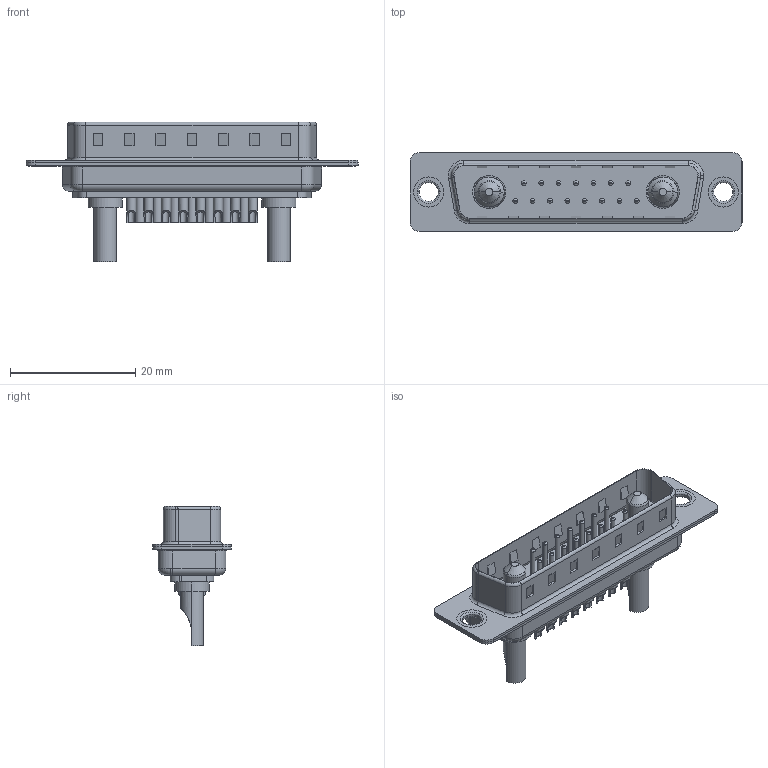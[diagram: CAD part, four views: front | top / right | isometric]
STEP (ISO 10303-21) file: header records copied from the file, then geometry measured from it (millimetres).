
FILE_DESCRIPTION (( 'STEP AP203' ), '1' );
FILE_NAME ('627-17W2222-2N1.STEP', '2019-05-27T14:13:00', ( '' ), ( '' ), 'SwSTEP 2.0', 'SolidWorks 2016', '' );
FILE_SCHEMA (( 'CONFIG_CONTROL_DESIGN' ));
Length unit declared in the file: millimetre
Products named in the file (8): 627Combo Contact Row 2_22; 627-17W2222-2N1; 627Combo Housing_17W2; 627Combo Shell Rear_25 Contacts; 627Combo Shell Front_25 Contacts; 627Combo Thru Hole Rivet; Power Pin_20A SC; 627Combo Contact Row 1_22
Assembly tree (22 placements, depth 2):
  627-17W2222-2N1
    627Combo Housing_17W2
    627Combo Shell Rear_25 Contacts
    627Combo Shell Front_25 Contacts
    627Combo Thru Hole Rivet  x2
    Power Pin_20A SC  x2
    627Combo Contact Row 1_22  x7
    627Combo Contact Row 2_22  x8
Bounding box: 53 x 12.6 x 22.3 mm (x, y, z)
Volume: 2826.9 mm3; surface area: 6927.3 mm2
Topology: 24 solids, 24 shells, 997 faces, 2339 edges, 1433 vertices
Faces by surface type: cylinder 405, plane 332, torus 212, cone 44, bspline 4
Entity records: 17934 total; most frequent: DIRECTION 3063, CARTESIAN_POINT 3025, ORIENTED_EDGE 2686, EDGE_CURVE 1343, AXIS2_PLACEMENT_3D 1181, VERTEX_POINT 849, LINE 701, VECTOR 701
